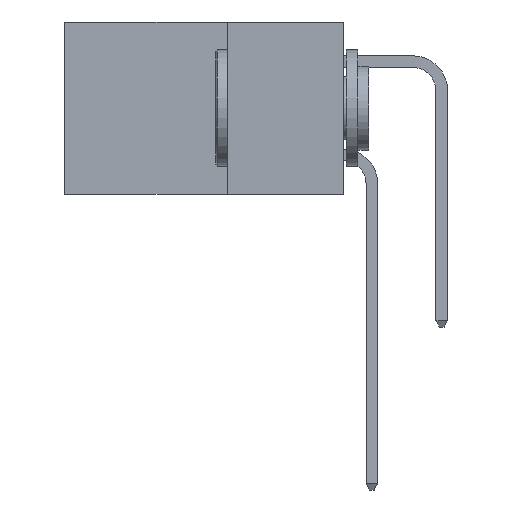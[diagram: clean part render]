
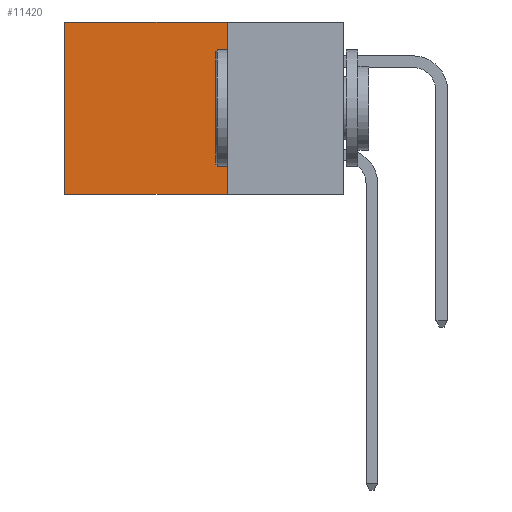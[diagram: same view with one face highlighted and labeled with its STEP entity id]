
A CAD part, left-side view. The second image highlights one B-rep face of the part: STEP entity #11420.
In plain terms, the highlighted planar face has unit normal (-1, 0, 0).
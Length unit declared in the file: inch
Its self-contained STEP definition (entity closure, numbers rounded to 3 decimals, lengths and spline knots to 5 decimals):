
#478 = VECTOR ( 'NONE', #9525, 39.37008 ) ;
#957 = EDGE_LOOP ( 'NONE', ( #10850, #6433, #6874, #4527 ) ) ;
#1528 = EDGE_CURVE ( 'NONE', #11397, #7771, #8933, .T. ) ;
#2673 = CARTESIAN_POINT ( 'NONE',  ( 0.2615, 0.25, -0.37 ) ) ;
#2814 = CARTESIAN_POINT ( 'NONE',  ( 0.2615, 0.6, -0.37 ) ) ;
#3339 = VERTEX_POINT ( 'NONE', #2814 ) ;
#3477 = CARTESIAN_POINT ( 'NONE',  ( 0.2615, 0.25, 0. ) ) ;
#3816 = DIRECTION ( 'NONE',  ( 0., 1., 0. ) ) ;
#3840 = CARTESIAN_POINT ( 'NONE',  ( 0.2615, 0.25, -0.37 ) ) ;
#3859 = CARTESIAN_POINT ( 'NONE',  ( 0.2615, 0.25, -0.37 ) ) ;
#4527 = ORIENTED_EDGE ( 'NONE', *, *, #1528, .T. ) ;
#4873 = VERTEX_POINT ( 'NONE', #2673 ) ;
#6308 = CARTESIAN_POINT ( 'NONE',  ( 0.2615, 0.6, -0.37 ) ) ;
#6433 = ORIENTED_EDGE ( 'NONE', *, *, #9061, .F. ) ;
#6551 = DIRECTION ( 'NONE',  ( 0., 0., -1. ) ) ;
#6623 = PLANE ( 'NONE',  #16763 ) ;
#6874 = ORIENTED_EDGE ( 'NONE', *, *, #18835, .F. ) ;
#6978 = VECTOR ( 'NONE', #6551, 39.37008 ) ;
#7771 = VERTEX_POINT ( 'NONE', #18857 ) ;
#7929 = VECTOR ( 'NONE', #12753, 39.37008 ) ;
#8089 = DIRECTION ( 'NONE',  ( 1., 0., 0. ) ) ;
#8815 = EDGE_CURVE ( 'NONE', #7771, #3339, #18258, .T. ) ;
#8933 = LINE ( 'NONE', #3477, #478 ) ;
#9061 = EDGE_CURVE ( 'NONE', #4873, #3339, #14428, .T. ) ;
#9459 = CARTESIAN_POINT ( 'NONE',  ( 0.2615, 0.25, 0. ) ) ;
#9525 = DIRECTION ( 'NONE',  ( 0., 1., 0. ) ) ;
#10850 = ORIENTED_EDGE ( 'NONE', *, *, #8815, .T. ) ;
#11397 = VERTEX_POINT ( 'NONE', #9459 ) ;
#11420 = ADVANCED_FACE ( 'NONE', ( #17413 ), #6623, .F. ) ;
#11885 = LINE ( 'NONE', #3859, #7929 ) ;
#12753 = DIRECTION ( 'NONE',  ( 0., 0., -1. ) ) ;
#14428 = LINE ( 'NONE', #3840, #18283 ) ;
#16763 = AXIS2_PLACEMENT_3D ( 'NONE', #16939, #8089, #18392 ) ;
#16939 = CARTESIAN_POINT ( 'NONE',  ( 0.2615, 0.25, -0.37 ) ) ;
#17413 = FACE_OUTER_BOUND ( 'NONE', #957, .T. ) ;
#18258 = LINE ( 'NONE', #6308, #6978 ) ;
#18283 = VECTOR ( 'NONE', #3816, 39.37008 ) ;
#18392 = DIRECTION ( 'NONE',  ( 0., 0., -1. ) ) ;
#18835 = EDGE_CURVE ( 'NONE', #11397, #4873, #11885, .T. ) ;
#18857 = CARTESIAN_POINT ( 'NONE',  ( 0.2615, 0.6, 0. ) ) ;
